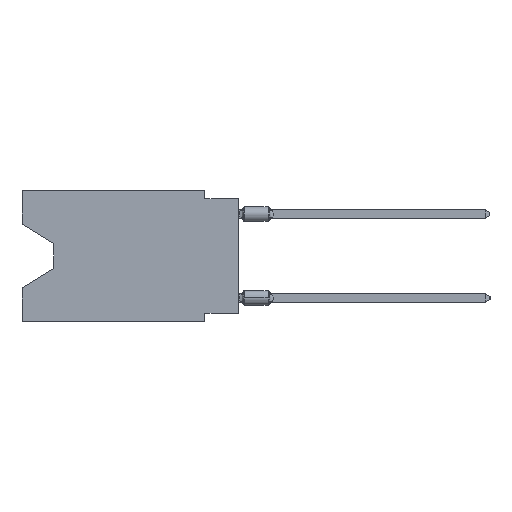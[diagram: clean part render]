
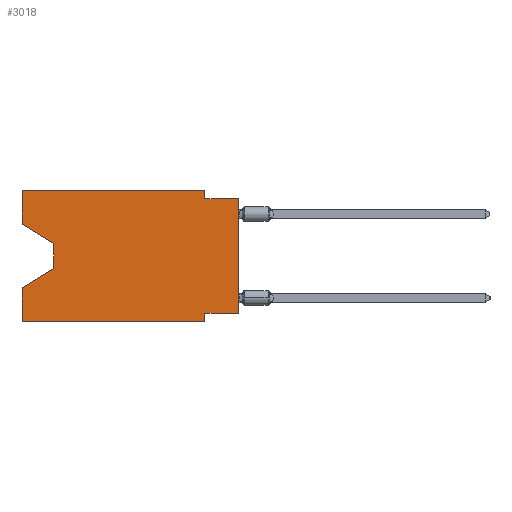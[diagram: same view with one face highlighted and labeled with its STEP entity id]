
A CAD part, left-side view. The second image highlights one B-rep face of the part: STEP entity #3018.
In plain terms, the highlighted planar face has unit normal (-1, 0, 0).
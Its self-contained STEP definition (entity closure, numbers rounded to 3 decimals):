
#52 = ORIENTED_EDGE ( 'NONE', *, *, #19327, .T. ) ;
#408 = DIRECTION ( 'NONE',  ( 0., -1., 0. ) ) ;
#1463 = CARTESIAN_POINT ( 'NONE',  ( 0., 2.54, -9.271 ) ) ;
#1712 = CARTESIAN_POINT ( 'NONE',  ( 0., 13.97, -5.893 ) ) ;
#2171 = EDGE_CURVE ( 'NONE', #32766, #11470, #32056, .T. ) ;
#2284 = LINE ( 'NONE', #32006, #23692 ) ;
#2559 = CARTESIAN_POINT ( 'NONE',  ( 0., 16.383, -9.906 ) ) ;
#3018 = ADVANCED_FACE ( 'NONE', ( #20801 ), #25526, .F. ) ;
#4385 = ORIENTED_EDGE ( 'NONE', *, *, #2171, .F. ) ;
#4753 = VERTEX_POINT ( 'NONE', #45137 ) ;
#5162 = DIRECTION ( 'NONE',  ( 0., 0., 1. ) ) ;
#5427 = ORIENTED_EDGE ( 'NONE', *, *, #27763, .F. ) ;
#5828 = ORIENTED_EDGE ( 'NONE', *, *, #28308, .T. ) ;
#5934 = EDGE_CURVE ( 'NONE', #12045, #9732, #40468, .T. ) ;
#5986 = ORIENTED_EDGE ( 'NONE', *, *, #19734, .F. ) ;
#6402 = ORIENTED_EDGE ( 'NONE', *, *, #27030, .F. ) ;
#6773 = VECTOR ( 'NONE', #34895, 1000. ) ;
#7435 = EDGE_CURVE ( 'NONE', #36568, #32766, #2284, .T. ) ;
#7644 = ORIENTED_EDGE ( 'NONE', *, *, #37202, .T. ) ;
#8337 = VECTOR ( 'NONE', #20729, 1000. ) ;
#9234 = CARTESIAN_POINT ( 'NONE',  ( 0., 0., -9.271 ) ) ;
#9732 = VERTEX_POINT ( 'NONE', #43083 ) ;
#10197 = DIRECTION ( 'NONE',  ( 1., 0., 0. ) ) ;
#11094 = CARTESIAN_POINT ( 'NONE',  ( 0., 0., 0. ) ) ;
#11451 = VECTOR ( 'NONE', #15441, 1000. ) ;
#11470 = VERTEX_POINT ( 'NONE', #18502 ) ;
#11637 = DIRECTION ( 'NONE',  ( 0., 0., 1. ) ) ;
#11721 = LINE ( 'NONE', #26110, #31399 ) ;
#12045 = VERTEX_POINT ( 'NONE', #2559 ) ;
#13016 = CARTESIAN_POINT ( 'NONE',  ( 0., 2.54, 0. ) ) ;
#13361 = VECTOR ( 'NONE', #5162, 1000. ) ;
#13943 = DIRECTION ( 'NONE',  ( 0., -1., 0. ) ) ;
#14448 = DIRECTION ( 'NONE',  ( 0., 0., -1. ) ) ;
#14567 = EDGE_CURVE ( 'NONE', #4753, #9732, #36868, .T. ) ;
#15441 = DIRECTION ( 'NONE',  ( 0., 0., -1. ) ) ;
#17203 = ORIENTED_EDGE ( 'NONE', *, *, #21516, .F. ) ;
#17262 = VERTEX_POINT ( 'NONE', #9234 ) ;
#17435 = LINE ( 'NONE', #24280, #8337 ) ;
#17629 = DIRECTION ( 'NONE',  ( 0., 0., -1. ) ) ;
#18058 = VECTOR ( 'NONE', #13943, 1000. ) ;
#18138 = DIRECTION ( 'NONE',  ( 0., -0.855, -0.519 ) ) ;
#18502 = CARTESIAN_POINT ( 'NONE',  ( 0., 0., -0.635 ) ) ;
#18719 = EDGE_CURVE ( 'NONE', #12045, #35549, #38943, .T. ) ;
#19327 = EDGE_CURVE ( 'NONE', #21116, #28584, #43815, .T. ) ;
#19734 = EDGE_CURVE ( 'NONE', #21116, #35379, #40180, .T. ) ;
#20061 = LINE ( 'NONE', #34445, #36679 ) ;
#20729 = DIRECTION ( 'NONE',  ( 0., 0., -1. ) ) ;
#20801 = FACE_OUTER_BOUND ( 'NONE', #42558, .T. ) ;
#21116 = VERTEX_POINT ( 'NONE', #22808 ) ;
#21225 = CARTESIAN_POINT ( 'NONE',  ( 0., 2.54, -0.635 ) ) ;
#21516 = EDGE_CURVE ( 'NONE', #30776, #35549, #44433, .T. ) ;
#22808 = CARTESIAN_POINT ( 'NONE',  ( 0., 16.383, -2.546 ) ) ;
#23692 = VECTOR ( 'NONE', #17629, 1000. ) ;
#24280 = CARTESIAN_POINT ( 'NONE',  ( 0., 13.97, -4.013 ) ) ;
#25526 = PLANE ( 'NONE',  #25603 ) ;
#25603 = AXIS2_PLACEMENT_3D ( 'NONE', #31647, #10197, #14448 ) ;
#26026 = DIRECTION ( 'NONE',  ( 0., 0.855, -0.519 ) ) ;
#26110 = CARTESIAN_POINT ( 'NONE',  ( 0., 16.383, 0. ) ) ;
#26314 = DIRECTION ( 'NONE',  ( 0., 0., 1. ) ) ;
#27030 = EDGE_CURVE ( 'NONE', #17262, #30776, #20061, .T. ) ;
#27763 = EDGE_CURVE ( 'NONE', #35379, #36568, #11721, .T. ) ;
#28166 = VECTOR ( 'NONE', #26314, 1000. ) ;
#28308 = EDGE_CURVE ( 'NONE', #17262, #11470, #43403, .T. ) ;
#28584 = VERTEX_POINT ( 'NONE', #36285 ) ;
#30776 = VERTEX_POINT ( 'NONE', #1463 ) ;
#30898 = DIRECTION ( 'NONE',  ( 0., 1., 0. ) ) ;
#31399 = VECTOR ( 'NONE', #408, 1000. ) ;
#31619 = CARTESIAN_POINT ( 'NONE',  ( 0., 16.383, -9.906 ) ) ;
#31647 = CARTESIAN_POINT ( 'NONE',  ( 0., 16.383, 0. ) ) ;
#32006 = CARTESIAN_POINT ( 'NONE',  ( 0., 2.54, 0. ) ) ;
#32056 = LINE ( 'NONE', #42198, #6773 ) ;
#32766 = VERTEX_POINT ( 'NONE', #21225 ) ;
#33146 = CARTESIAN_POINT ( 'NONE',  ( 0., 16.383, 0. ) ) ;
#33681 = ORIENTED_EDGE ( 'NONE', *, *, #5934, .F. ) ;
#33812 = CARTESIAN_POINT ( 'NONE',  ( 0., 2.54, -9.906 ) ) ;
#34445 = CARTESIAN_POINT ( 'NONE',  ( 0., 0., -9.271 ) ) ;
#34665 = VECTOR ( 'NONE', #26026, 1000. ) ;
#34895 = DIRECTION ( 'NONE',  ( 0., -1., 0. ) ) ;
#35266 = ORIENTED_EDGE ( 'NONE', *, *, #7435, .F. ) ;
#35379 = VERTEX_POINT ( 'NONE', #37997 ) ;
#35549 = VERTEX_POINT ( 'NONE', #40753 ) ;
#36171 = VECTOR ( 'NONE', #18138, 1000. ) ;
#36215 = VECTOR ( 'NONE', #11637, 1000. ) ;
#36285 = CARTESIAN_POINT ( 'NONE',  ( 0., 13.97, -4.013 ) ) ;
#36297 = CARTESIAN_POINT ( 'NONE',  ( 0., 16.383, -2.546 ) ) ;
#36568 = VERTEX_POINT ( 'NONE', #13016 ) ;
#36679 = VECTOR ( 'NONE', #30898, 1000. ) ;
#36868 = LINE ( 'NONE', #1712, #34665 ) ;
#37202 = EDGE_CURVE ( 'NONE', #28584, #4753, #17435, .T. ) ;
#37747 = ORIENTED_EDGE ( 'NONE', *, *, #18719, .T. ) ;
#37997 = CARTESIAN_POINT ( 'NONE',  ( 0., 16.383, 0. ) ) ;
#38691 = ORIENTED_EDGE ( 'NONE', *, *, #14567, .T. ) ;
#38943 = LINE ( 'NONE', #31619, #18058 ) ;
#40180 = LINE ( 'NONE', #43938, #36215 ) ;
#40468 = LINE ( 'NONE', #33146, #28166 ) ;
#40753 = CARTESIAN_POINT ( 'NONE',  ( 0., 2.54, -9.906 ) ) ;
#42198 = CARTESIAN_POINT ( 'NONE',  ( 0., 0., -0.635 ) ) ;
#42558 = EDGE_LOOP ( 'NONE', ( #52, #7644, #38691, #33681, #37747, #17203, #6402, #5828, #4385, #35266, #5427, #5986 ) ) ;
#43083 = CARTESIAN_POINT ( 'NONE',  ( 0., 16.383, -7.36 ) ) ;
#43403 = LINE ( 'NONE', #11094, #13361 ) ;
#43815 = LINE ( 'NONE', #36297, #36171 ) ;
#43938 = CARTESIAN_POINT ( 'NONE',  ( 0., 16.383, 0. ) ) ;
#44433 = LINE ( 'NONE', #33812, #11451 ) ;
#45137 = CARTESIAN_POINT ( 'NONE',  ( 0., 13.97, -5.893 ) ) ;
